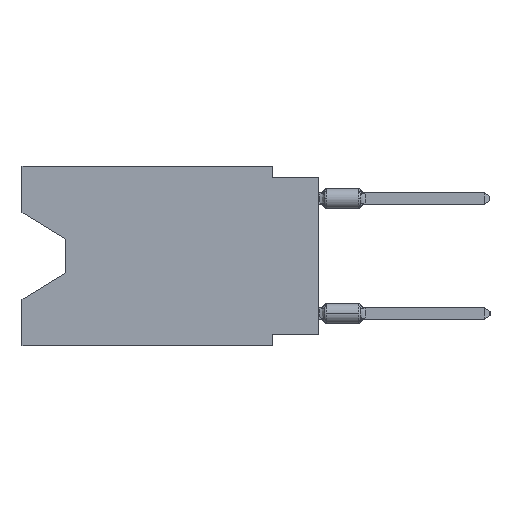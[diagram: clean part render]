
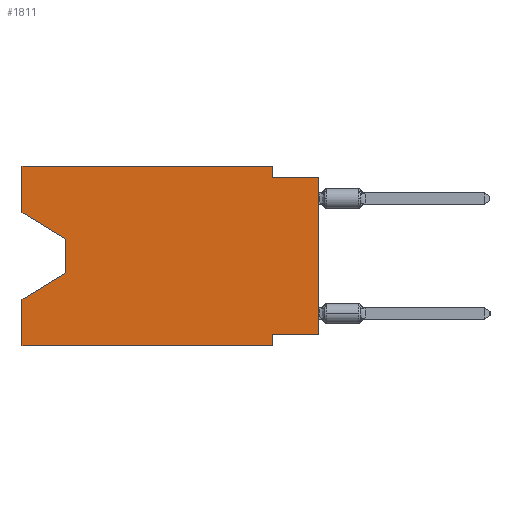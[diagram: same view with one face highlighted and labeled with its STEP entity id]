
A CAD part, left-side view. The second image highlights one B-rep face of the part: STEP entity #1811.
In plain terms, the highlighted planar face has unit normal (-1, 0, 0).
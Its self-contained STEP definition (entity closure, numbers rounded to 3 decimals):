
#296 = DIRECTION ( 'NONE',  ( 0., 0.855, -0.519 ) ) ;
#476 = LINE ( 'NONE', #3163, #26646 ) ;
#1236 = CARTESIAN_POINT ( 'NONE',  ( 0., 2.54, -0.635 ) ) ;
#1811 = ADVANCED_FACE ( 'NONE', ( #7717 ), #21688, .F. ) ;
#1852 = CARTESIAN_POINT ( 'NONE',  ( 0., 13.97, -4.013 ) ) ;
#1853 = EDGE_CURVE ( 'NONE', #31458, #9855, #20060, .T. ) ;
#2267 = LINE ( 'NONE', #18746, #3141 ) ;
#2472 = ORIENTED_EDGE ( 'NONE', *, *, #15992, .F. ) ;
#2473 = ORIENTED_EDGE ( 'NONE', *, *, #22082, .T. ) ;
#3117 = CARTESIAN_POINT ( 'NONE',  ( 0., 2.54, -9.906 ) ) ;
#3141 = VECTOR ( 'NONE', #8168, 1000. ) ;
#3163 = CARTESIAN_POINT ( 'NONE',  ( 0., 13.97, -4.013 ) ) ;
#4464 = VERTEX_POINT ( 'NONE', #32507 ) ;
#5093 = DIRECTION ( 'NONE',  ( 0., 0., -1. ) ) ;
#6727 = EDGE_CURVE ( 'NONE', #22164, #16637, #476, .T. ) ;
#7142 = ORIENTED_EDGE ( 'NONE', *, *, #30798, .F. ) ;
#7717 = FACE_OUTER_BOUND ( 'NONE', #32977, .T. ) ;
#8158 = DIRECTION ( 'NONE',  ( 0., 0., 1. ) ) ;
#8168 = DIRECTION ( 'NONE',  ( 0., -1., 0. ) ) ;
#8419 = CARTESIAN_POINT ( 'NONE',  ( 0., 16.383, -2.546 ) ) ;
#8437 = VECTOR ( 'NONE', #31726, 1000. ) ;
#8753 = VERTEX_POINT ( 'NONE', #9332 ) ;
#8970 = CARTESIAN_POINT ( 'NONE',  ( 0., 16.383, -9.906 ) ) ;
#9186 = VECTOR ( 'NONE', #10452, 1000. ) ;
#9332 = CARTESIAN_POINT ( 'NONE',  ( 0., 0., -0.635 ) ) ;
#9508 = ORIENTED_EDGE ( 'NONE', *, *, #6727, .T. ) ;
#9855 = VERTEX_POINT ( 'NONE', #34648 ) ;
#10247 = LINE ( 'NONE', #29032, #27637 ) ;
#10452 = DIRECTION ( 'NONE',  ( 0., 0., 1. ) ) ;
#10493 = EDGE_CURVE ( 'NONE', #4464, #9855, #11539, .T. ) ;
#11539 = LINE ( 'NONE', #3117, #34475 ) ;
#11765 = EDGE_CURVE ( 'NONE', #16637, #14389, #19649, .T. ) ;
#11891 = CARTESIAN_POINT ( 'NONE',  ( 0., 16.383, 0. ) ) ;
#12028 = ORIENTED_EDGE ( 'NONE', *, *, #11765, .T. ) ;
#12356 = EDGE_CURVE ( 'NONE', #26457, #4464, #24176, .T. ) ;
#12359 = ORIENTED_EDGE ( 'NONE', *, *, #12356, .F. ) ;
#13928 = VECTOR ( 'NONE', #30956, 1000. ) ;
#14095 = DIRECTION ( 'NONE',  ( 0., 0., -1. ) ) ;
#14141 = VERTEX_POINT ( 'NONE', #22341 ) ;
#14314 = CARTESIAN_POINT ( 'NONE',  ( 0., 0., -9.271 ) ) ;
#14389 = VERTEX_POINT ( 'NONE', #34604 ) ;
#14890 = VERTEX_POINT ( 'NONE', #29554 ) ;
#15143 = VERTEX_POINT ( 'NONE', #1236 ) ;
#15433 = DIRECTION ( 'NONE',  ( 0., -1., 0. ) ) ;
#15623 = AXIS2_PLACEMENT_3D ( 'NONE', #24027, #29902, #34922 ) ;
#15992 = EDGE_CURVE ( 'NONE', #14890, #15143, #25655, .T. ) ;
#16637 = VERTEX_POINT ( 'NONE', #23580 ) ;
#17251 = EDGE_CURVE ( 'NONE', #31458, #14389, #31003, .T. ) ;
#17361 = EDGE_CURVE ( 'NONE', #14141, #14890, #10247, .T. ) ;
#17390 = ORIENTED_EDGE ( 'NONE', *, *, #17361, .F. ) ;
#18480 = VECTOR ( 'NONE', #25491, 1000. ) ;
#18746 = CARTESIAN_POINT ( 'NONE',  ( 0., 0., -0.635 ) ) ;
#19366 = VERTEX_POINT ( 'NONE', #8419 ) ;
#19649 = LINE ( 'NONE', #35225, #31102 ) ;
#20060 = LINE ( 'NONE', #8970, #13928 ) ;
#20812 = CARTESIAN_POINT ( 'NONE',  ( 0., 16.383, -2.546 ) ) ;
#20813 = CARTESIAN_POINT ( 'NONE',  ( 0., 16.383, -9.906 ) ) ;
#21688 = PLANE ( 'NONE',  #15623 ) ;
#22082 = EDGE_CURVE ( 'NONE', #26457, #8753, #34972, .T. ) ;
#22164 = VERTEX_POINT ( 'NONE', #1852 ) ;
#22341 = CARTESIAN_POINT ( 'NONE',  ( 0., 16.383, 0. ) ) ;
#22381 = DIRECTION ( 'NONE',  ( 0., 1., 0. ) ) ;
#22603 = VECTOR ( 'NONE', #22381, 1000. ) ;
#22694 = VECTOR ( 'NONE', #5093, 1000. ) ;
#22981 = LINE ( 'NONE', #20812, #8437 ) ;
#23351 = CARTESIAN_POINT ( 'NONE',  ( 0., 0., -9.271 ) ) ;
#23580 = CARTESIAN_POINT ( 'NONE',  ( 0., 13.97, -5.893 ) ) ;
#23703 = EDGE_CURVE ( 'NONE', #19366, #22164, #22981, .T. ) ;
#23746 = ORIENTED_EDGE ( 'NONE', *, *, #23703, .T. ) ;
#24027 = CARTESIAN_POINT ( 'NONE',  ( 0., 16.383, 0. ) ) ;
#24176 = LINE ( 'NONE', #14314, #22603 ) ;
#25491 = DIRECTION ( 'NONE',  ( 0., 0., 1. ) ) ;
#25655 = LINE ( 'NONE', #35181, #22694 ) ;
#25684 = ORIENTED_EDGE ( 'NONE', *, *, #1853, .T. ) ;
#26457 = VERTEX_POINT ( 'NONE', #23351 ) ;
#26646 = VECTOR ( 'NONE', #14095, 1000. ) ;
#26932 = CARTESIAN_POINT ( 'NONE',  ( 0., 0., 0. ) ) ;
#27330 = CARTESIAN_POINT ( 'NONE',  ( 0., 16.383, 0. ) ) ;
#27637 = VECTOR ( 'NONE', #15433, 1000. ) ;
#29032 = CARTESIAN_POINT ( 'NONE',  ( 0., 16.383, 0. ) ) ;
#29157 = EDGE_CURVE ( 'NONE', #19366, #14141, #29814, .T. ) ;
#29554 = CARTESIAN_POINT ( 'NONE',  ( 0., 2.54, 0. ) ) ;
#29814 = LINE ( 'NONE', #27330, #34010 ) ;
#29902 = DIRECTION ( 'NONE',  ( 1., 0., 0. ) ) ;
#30329 = DIRECTION ( 'NONE',  ( 0., 0., -1. ) ) ;
#30335 = ORIENTED_EDGE ( 'NONE', *, *, #17251, .F. ) ;
#30798 = EDGE_CURVE ( 'NONE', #15143, #8753, #2267, .T. ) ;
#30956 = DIRECTION ( 'NONE',  ( 0., -1., 0. ) ) ;
#30969 = ORIENTED_EDGE ( 'NONE', *, *, #29157, .F. ) ;
#31003 = LINE ( 'NONE', #11891, #18480 ) ;
#31102 = VECTOR ( 'NONE', #296, 1000. ) ;
#31458 = VERTEX_POINT ( 'NONE', #20813 ) ;
#31726 = DIRECTION ( 'NONE',  ( 0., -0.855, -0.519 ) ) ;
#32507 = CARTESIAN_POINT ( 'NONE',  ( 0., 2.54, -9.271 ) ) ;
#32935 = ORIENTED_EDGE ( 'NONE', *, *, #10493, .F. ) ;
#32977 = EDGE_LOOP ( 'NONE', ( #23746, #9508, #12028, #30335, #25684, #32935, #12359, #2473, #7142, #2472, #17390, #30969 ) ) ;
#34010 = VECTOR ( 'NONE', #8158, 1000. ) ;
#34475 = VECTOR ( 'NONE', #30329, 1000. ) ;
#34604 = CARTESIAN_POINT ( 'NONE',  ( 0., 16.383, -7.36 ) ) ;
#34648 = CARTESIAN_POINT ( 'NONE',  ( 0., 2.54, -9.906 ) ) ;
#34922 = DIRECTION ( 'NONE',  ( 0., 0., -1. ) ) ;
#34972 = LINE ( 'NONE', #26932, #9186 ) ;
#35181 = CARTESIAN_POINT ( 'NONE',  ( 0., 2.54, 0. ) ) ;
#35225 = CARTESIAN_POINT ( 'NONE',  ( 0., 13.97, -5.893 ) ) ;
